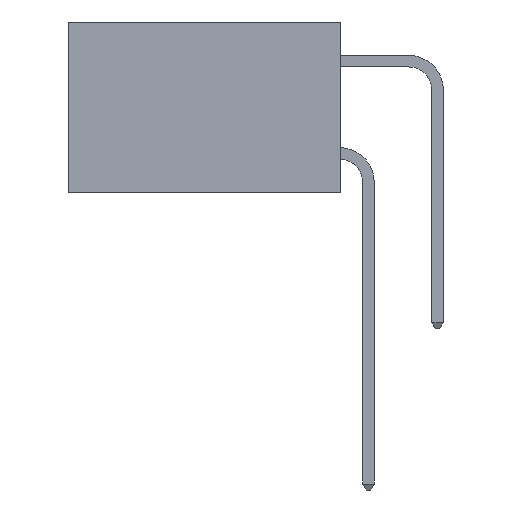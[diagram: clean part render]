
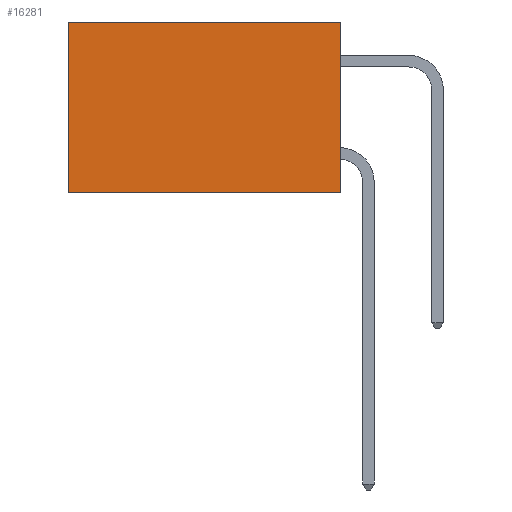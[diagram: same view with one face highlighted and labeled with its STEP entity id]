
A CAD part, left-side view. The second image highlights one B-rep face of the part: STEP entity #16281.
In plain terms, the highlighted planar face has unit normal (-1, 0, 0).
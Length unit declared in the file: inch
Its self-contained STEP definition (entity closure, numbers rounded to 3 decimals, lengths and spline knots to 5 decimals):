
#712 = DIRECTION ( 'NONE',  ( 0., 1., 0. ) ) ;
#760 = VERTEX_POINT ( 'NONE', #7511 ) ;
#898 = VECTOR ( 'NONE', #12371, 39.37008 ) ;
#921 = DIRECTION ( 'NONE',  ( 0., 0., -1. ) ) ;
#1492 = CARTESIAN_POINT ( 'NONE',  ( 0.277, 0.59, -0.37 ) ) ;
#1795 = CARTESIAN_POINT ( 'NONE',  ( 0.277, 0., -0.37 ) ) ;
#1928 = EDGE_CURVE ( 'NONE', #760, #17445, #15397, .T. ) ;
#2019 = PLANE ( 'NONE',  #4936 ) ;
#2123 = CARTESIAN_POINT ( 'NONE',  ( 0.277, 0., -0.37 ) ) ;
#2740 = CARTESIAN_POINT ( 'NONE',  ( 0.277, 0., 0. ) ) ;
#3210 = VECTOR ( 'NONE', #4559, 39.37008 ) ;
#4230 = ORIENTED_EDGE ( 'NONE', *, *, #1928, .F. ) ;
#4492 = FACE_OUTER_BOUND ( 'NONE', #6285, .T. ) ;
#4559 = DIRECTION ( 'NONE',  ( 0., 0., -1. ) ) ;
#4630 = ORIENTED_EDGE ( 'NONE', *, *, #12370, .T. ) ;
#4692 = ORIENTED_EDGE ( 'NONE', *, *, #16887, .F. ) ;
#4822 = DIRECTION ( 'NONE',  ( 1., 0., 0. ) ) ;
#4917 = ORIENTED_EDGE ( 'NONE', *, *, #15479, .T. ) ;
#4936 = AXIS2_PLACEMENT_3D ( 'NONE', #13012, #4822, #14348 ) ;
#5210 = VERTEX_POINT ( 'NONE', #9213 ) ;
#6285 = EDGE_LOOP ( 'NONE', ( #4917, #4692, #4230, #4630 ) ) ;
#7511 = CARTESIAN_POINT ( 'NONE',  ( 0.277, 0., 0. ) ) ;
#9213 = CARTESIAN_POINT ( 'NONE',  ( 0.277, 0.59, 0. ) ) ;
#9599 = LINE ( 'NONE', #2123, #15951 ) ;
#11827 = VECTOR ( 'NONE', #921, 39.37008 ) ;
#12370 = EDGE_CURVE ( 'NONE', #760, #5210, #14642, .T. ) ;
#12371 = DIRECTION ( 'NONE',  ( 0., 1., 0. ) ) ;
#12741 = LINE ( 'NONE', #16754, #3210 ) ;
#12942 = CARTESIAN_POINT ( 'NONE',  ( 0.277, 0., -0.37 ) ) ;
#13012 = CARTESIAN_POINT ( 'NONE',  ( 0.277, 0., -0.37 ) ) ;
#14348 = DIRECTION ( 'NONE',  ( 0., 0., -1. ) ) ;
#14642 = LINE ( 'NONE', #2740, #898 ) ;
#15356 = VERTEX_POINT ( 'NONE', #1492 ) ;
#15397 = LINE ( 'NONE', #12942, #11827 ) ;
#15479 = EDGE_CURVE ( 'NONE', #5210, #15356, #12741, .T. ) ;
#15951 = VECTOR ( 'NONE', #712, 39.37008 ) ;
#16281 = ADVANCED_FACE ( 'NONE', ( #4492 ), #2019, .F. ) ;
#16754 = CARTESIAN_POINT ( 'NONE',  ( 0.277, 0.59, -0.37 ) ) ;
#16887 = EDGE_CURVE ( 'NONE', #17445, #15356, #9599, .T. ) ;
#17445 = VERTEX_POINT ( 'NONE', #1795 ) ;
